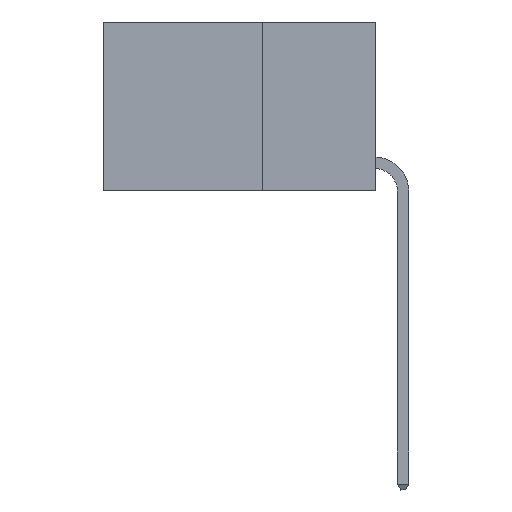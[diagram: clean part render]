
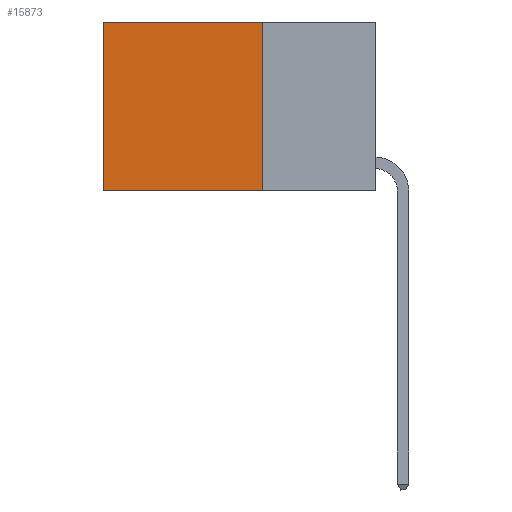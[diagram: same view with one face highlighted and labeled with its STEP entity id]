
A CAD part, left-side view. The second image highlights one B-rep face of the part: STEP entity #15873.
In plain terms, the highlighted planar face has unit normal (-1, 0, 0).
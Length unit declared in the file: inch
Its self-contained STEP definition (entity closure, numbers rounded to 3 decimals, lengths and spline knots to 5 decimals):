
#1281 = CARTESIAN_POINT ( 'NONE',  ( 0.2625, 0.25, -0.37 ) ) ;
#2349 = DIRECTION ( 'NONE',  ( 0., 0., -1. ) ) ;
#3449 = DIRECTION ( 'NONE',  ( 0., 0., -1. ) ) ;
#4326 = DIRECTION ( 'NONE',  ( 0., 0., -1. ) ) ;
#4487 = DIRECTION ( 'NONE',  ( 1., 0., 0. ) ) ;
#5740 = VERTEX_POINT ( 'NONE', #6771 ) ;
#5874 = EDGE_CURVE ( 'NONE', #9122, #5740, #11515, .T. ) ;
#5937 = ORIENTED_EDGE ( 'NONE', *, *, #7974, .T. ) ;
#6404 = DIRECTION ( 'NONE',  ( 0., 1., 0. ) ) ;
#6771 = CARTESIAN_POINT ( 'NONE',  ( 0.2625, 0.6, -0.37 ) ) ;
#6992 = LINE ( 'NONE', #9668, #11821 ) ;
#7393 = EDGE_CURVE ( 'NONE', #15523, #5740, #12886, .T. ) ;
#7548 = CARTESIAN_POINT ( 'NONE',  ( 0.2625, 0.25, 0. ) ) ;
#7680 = VECTOR ( 'NONE', #2349, 39.37008 ) ;
#7974 = EDGE_CURVE ( 'NONE', #12379, #9122, #13515, .T. ) ;
#8469 = CARTESIAN_POINT ( 'NONE',  ( 0.2625, 0.6, 0. ) ) ;
#9122 = VERTEX_POINT ( 'NONE', #8469 ) ;
#9668 = CARTESIAN_POINT ( 'NONE',  ( 0.2625, 0.25, 0. ) ) ;
#10512 = ORIENTED_EDGE ( 'NONE', *, *, #11777, .F. ) ;
#10744 = CARTESIAN_POINT ( 'NONE',  ( 0.2625, 0.25, 0. ) ) ;
#11515 = LINE ( 'NONE', #16435, #7680 ) ;
#11777 = EDGE_CURVE ( 'NONE', #12379, #15523, #6992, .T. ) ;
#11821 = VECTOR ( 'NONE', #3449, 39.37008 ) ;
#11962 = CARTESIAN_POINT ( 'NONE',  ( 0.2625, 0.25, 0. ) ) ;
#12209 = PLANE ( 'NONE',  #14371 ) ;
#12379 = VERTEX_POINT ( 'NONE', #7548 ) ;
#12886 = LINE ( 'NONE', #1281, #14159 ) ;
#13204 = EDGE_LOOP ( 'NONE', ( #15202, #15859, #10512, #5937 ) ) ;
#13515 = LINE ( 'NONE', #10744, #15541 ) ;
#14159 = VECTOR ( 'NONE', #6404, 39.37008 ) ;
#14371 = AXIS2_PLACEMENT_3D ( 'NONE', #11962, #4487, #4326 ) ;
#14673 = FACE_OUTER_BOUND ( 'NONE', #13204, .T. ) ;
#15202 = ORIENTED_EDGE ( 'NONE', *, *, #5874, .T. ) ;
#15523 = VERTEX_POINT ( 'NONE', #16290 ) ;
#15541 = VECTOR ( 'NONE', #15904, 39.37008 ) ;
#15859 = ORIENTED_EDGE ( 'NONE', *, *, #7393, .F. ) ;
#15873 = ADVANCED_FACE ( 'NONE', ( #14673 ), #12209, .F. ) ;
#15904 = DIRECTION ( 'NONE',  ( 0., 1., 0. ) ) ;
#16290 = CARTESIAN_POINT ( 'NONE',  ( 0.2625, 0.25, -0.37 ) ) ;
#16435 = CARTESIAN_POINT ( 'NONE',  ( 0.2625, 0.6, 0. ) ) ;
